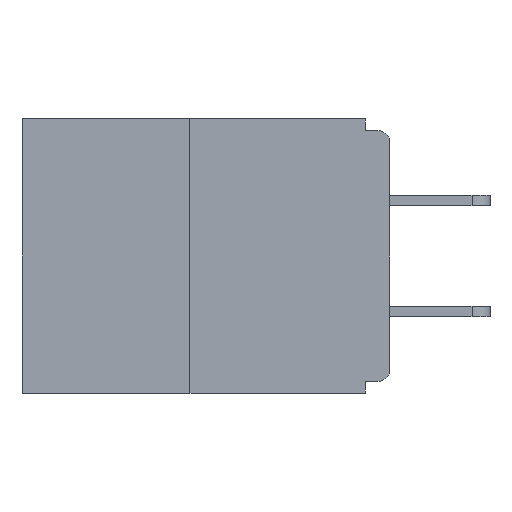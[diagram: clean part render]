
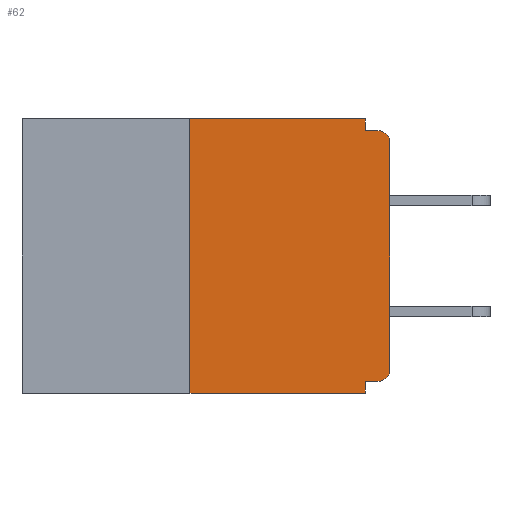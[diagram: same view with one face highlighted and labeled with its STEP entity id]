
A CAD part, left-side view. The second image highlights one B-rep face of the part: STEP entity #62.
In plain terms, the highlighted planar face has unit normal (-1, 0, 0).
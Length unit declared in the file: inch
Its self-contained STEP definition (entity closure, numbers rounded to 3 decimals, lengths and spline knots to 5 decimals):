
#62 = ADVANCED_FACE ( 'NONE', ( #20713 ), #14494, .F. ) ;
#190 = ORIENTED_EDGE ( 'NONE', *, *, #20895, .F. ) ;
#233 = CARTESIAN_POINT ( 'NONE',  ( 0., 0.25, 0. ) ) ;
#829 = CIRCLE ( 'NONE', #17938, 0.015 ) ;
#1388 = DIRECTION ( 'NONE',  ( 0., 0., -1. ) ) ;
#1460 = CARTESIAN_POINT ( 'NONE',  ( 0., 0., -0.015 ) ) ;
#1807 = EDGE_CURVE ( 'NONE', #17889, #12966, #3434, .T. ) ;
#2446 = DIRECTION ( 'NONE',  ( 0., 0., -1. ) ) ;
#2674 = VERTEX_POINT ( 'NONE', #22921 ) ;
#3434 = LINE ( 'NONE', #22221, #7126 ) ;
#3596 = DIRECTION ( 'NONE',  ( 0., -1., 0. ) ) ;
#3733 = ORIENTED_EDGE ( 'NONE', *, *, #15827, .F. ) ;
#4216 = ORIENTED_EDGE ( 'NONE', *, *, #21983, .T. ) ;
#4339 = LINE ( 'NONE', #21853, #13669 ) ;
#4698 = ORIENTED_EDGE ( 'NONE', *, *, #1807, .T. ) ;
#4788 = EDGE_CURVE ( 'NONE', #11156, #13106, #9394, .T. ) ;
#5177 = DIRECTION ( 'NONE',  ( 0., 0., -1. ) ) ;
#5515 = VECTOR ( 'NONE', #2446, 39.37008 ) ;
#5615 = ORIENTED_EDGE ( 'NONE', *, *, #10306, .T. ) ;
#5774 = AXIS2_PLACEMENT_3D ( 'NONE', #12391, #14204, #5177 ) ;
#6382 = CARTESIAN_POINT ( 'NONE',  ( 0., 0.031, 0. ) ) ;
#6545 = CARTESIAN_POINT ( 'NONE',  ( 0., 0., -0.313 ) ) ;
#7126 = VECTOR ( 'NONE', #15031, 39.37008 ) ;
#7311 = DIRECTION ( 'NONE',  ( 0., 0., -1. ) ) ;
#7467 = VERTEX_POINT ( 'NONE', #22073 ) ;
#7874 = EDGE_LOOP ( 'NONE', ( #3733, #190, #14481, #11446, #21299, #4216, #4698, #5615, #9465, #13239 ) ) ;
#8297 = DIRECTION ( 'NONE',  ( 0., -1., 0. ) ) ;
#9070 = CARTESIAN_POINT ( 'NONE',  ( 0., 0., -0.328 ) ) ;
#9076 = EDGE_CURVE ( 'NONE', #21937, #11156, #19670, .T. ) ;
#9126 = VECTOR ( 'NONE', #19943, 39.37008 ) ;
#9304 = DIRECTION ( 'NONE',  ( 0., -1., 0. ) ) ;
#9394 = LINE ( 'NONE', #10523, #18448 ) ;
#9465 = ORIENTED_EDGE ( 'NONE', *, *, #10423, .F. ) ;
#10253 = CIRCLE ( 'NONE', #5774, 0.015 ) ;
#10306 = EDGE_CURVE ( 'NONE', #12966, #2674, #10253, .T. ) ;
#10344 = LINE ( 'NONE', #13068, #5515 ) ;
#10423 = EDGE_CURVE ( 'NONE', #7467, #2674, #13061, .T. ) ;
#10516 = DIRECTION ( 'NONE',  ( -1., 0., 0. ) ) ;
#10523 = CARTESIAN_POINT ( 'NONE',  ( 0., 0.031, -0.343 ) ) ;
#10881 = DIRECTION ( 'NONE',  ( 0., 1., 0. ) ) ;
#11156 = VERTEX_POINT ( 'NONE', #16020 ) ;
#11446 = ORIENTED_EDGE ( 'NONE', *, *, #4788, .F. ) ;
#12071 = CARTESIAN_POINT ( 'NONE',  ( 0., 0.46, 0. ) ) ;
#12124 = CARTESIAN_POINT ( 'NONE',  ( 0., 0.25, 0. ) ) ;
#12391 = CARTESIAN_POINT ( 'NONE',  ( 0., 0.015, -0.03 ) ) ;
#12607 = CARTESIAN_POINT ( 'NONE',  ( 0., 0.46, 0. ) ) ;
#12608 = LINE ( 'NONE', #12071, #17392 ) ;
#12788 = CARTESIAN_POINT ( 'NONE',  ( 0., 0.031, -0.343 ) ) ;
#12966 = VERTEX_POINT ( 'NONE', #14438 ) ;
#13061 = LINE ( 'NONE', #1460, #15869 ) ;
#13068 = CARTESIAN_POINT ( 'NONE',  ( 0., 0.031, 0. ) ) ;
#13106 = VERTEX_POINT ( 'NONE', #12788 ) ;
#13239 = ORIENTED_EDGE ( 'NONE', *, *, #14264, .F. ) ;
#13669 = VECTOR ( 'NONE', #9304, 39.37008 ) ;
#13933 = VERTEX_POINT ( 'NONE', #12124 ) ;
#14204 = DIRECTION ( 'NONE',  ( -1., 0., 0. ) ) ;
#14264 = EDGE_CURVE ( 'NONE', #18000, #7467, #10344, .T. ) ;
#14438 = CARTESIAN_POINT ( 'NONE',  ( 0., 0., -0.03 ) ) ;
#14481 = ORIENTED_EDGE ( 'NONE', *, *, #15192, .T. ) ;
#14494 = PLANE ( 'NONE',  #15197 ) ;
#15031 = DIRECTION ( 'NONE',  ( 0., 0., 1. ) ) ;
#15192 = EDGE_CURVE ( 'NONE', #17117, #13106, #4339, .T. ) ;
#15197 = AXIS2_PLACEMENT_3D ( 'NONE', #12607, #16319, #7311 ) ;
#15827 = EDGE_CURVE ( 'NONE', #13933, #18000, #12608, .T. ) ;
#15869 = VECTOR ( 'NONE', #3596, 39.37008 ) ;
#16020 = CARTESIAN_POINT ( 'NONE',  ( 0., 0.031, -0.328 ) ) ;
#16319 = DIRECTION ( 'NONE',  ( 1., 0., 0. ) ) ;
#17117 = VERTEX_POINT ( 'NONE', #19190 ) ;
#17392 = VECTOR ( 'NONE', #8297, 39.37008 ) ;
#17889 = VERTEX_POINT ( 'NONE', #6545 ) ;
#17938 = AXIS2_PLACEMENT_3D ( 'NONE', #19661, #10516, #23157 ) ;
#18000 = VERTEX_POINT ( 'NONE', #6382 ) ;
#18448 = VECTOR ( 'NONE', #1388, 39.37008 ) ;
#19190 = CARTESIAN_POINT ( 'NONE',  ( 0., 0.25, -0.343 ) ) ;
#19661 = CARTESIAN_POINT ( 'NONE',  ( 0., 0.015, -0.313 ) ) ;
#19670 = LINE ( 'NONE', #9070, #20217 ) ;
#19943 = DIRECTION ( 'NONE',  ( 0., 0., 1. ) ) ;
#20217 = VECTOR ( 'NONE', #10881, 39.37008 ) ;
#20713 = FACE_OUTER_BOUND ( 'NONE', #7874, .T. ) ;
#20895 = EDGE_CURVE ( 'NONE', #17117, #13933, #21558, .T. ) ;
#21299 = ORIENTED_EDGE ( 'NONE', *, *, #9076, .F. ) ;
#21471 = CARTESIAN_POINT ( 'NONE',  ( 0., 0.015, -0.328 ) ) ;
#21558 = LINE ( 'NONE', #233, #9126 ) ;
#21853 = CARTESIAN_POINT ( 'NONE',  ( 0., 0.46, -0.343 ) ) ;
#21937 = VERTEX_POINT ( 'NONE', #21471 ) ;
#21983 = EDGE_CURVE ( 'NONE', #21937, #17889, #829, .T. ) ;
#22073 = CARTESIAN_POINT ( 'NONE',  ( 0., 0.031, -0.015 ) ) ;
#22221 = CARTESIAN_POINT ( 'NONE',  ( 0., 0., 0. ) ) ;
#22921 = CARTESIAN_POINT ( 'NONE',  ( 0., 0.015, -0.015 ) ) ;
#23157 = DIRECTION ( 'NONE',  ( 0., 0., -1. ) ) ;
